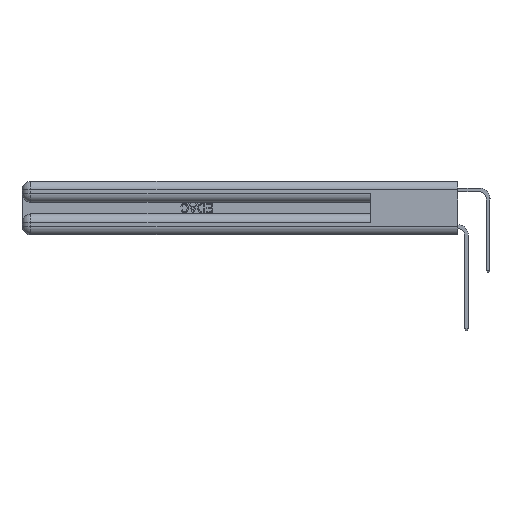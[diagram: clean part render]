
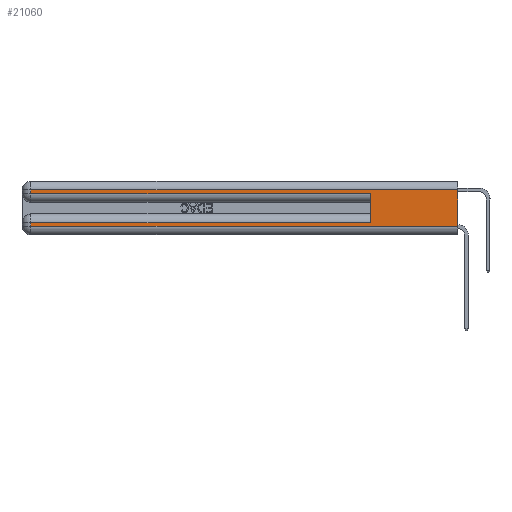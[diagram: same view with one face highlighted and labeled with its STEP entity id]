
A CAD part, left-side view. The second image highlights one B-rep face of the part: STEP entity #21060.
In plain terms, the highlighted planar face has unit normal (-1, 0, 0).
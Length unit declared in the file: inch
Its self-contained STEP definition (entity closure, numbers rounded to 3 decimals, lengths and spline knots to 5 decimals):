
#535 = DIRECTION ( 'NONE',  ( 0., 0., -1. ) ) ;
#800 = ORIENTED_EDGE ( 'NONE', *, *, #20794, .T. ) ;
#1014 = AXIS2_PLACEMENT_3D ( 'NONE', #16914, #11546, #22222 ) ;
#1233 = VECTOR ( 'NONE', #24987, 39.37008 ) ;
#1885 = ORIENTED_EDGE ( 'NONE', *, *, #12425, .F. ) ;
#2637 = VECTOR ( 'NONE', #28939, 39.37008 ) ;
#2693 = CARTESIAN_POINT ( 'NONE',  ( 0., 2.94, 0.06 ) ) ;
#4234 = CARTESIAN_POINT ( 'NONE',  ( 0., 0.6, 0.285 ) ) ;
#4418 = VERTEX_POINT ( 'NONE', #12762 ) ;
#4594 = LINE ( 'NONE', #8954, #20139 ) ;
#5728 = LINE ( 'NONE', #24723, #25001 ) ;
#6314 = LINE ( 'NONE', #26965, #32523 ) ;
#6561 = EDGE_LOOP ( 'NONE', ( #26309, #16931, #18086, #800, #1885, #12907, #27303, #20859 ) ) ;
#7468 = VERTEX_POINT ( 'NONE', #22239 ) ;
#8585 = LINE ( 'NONE', #22189, #1233 ) ;
#8954 = CARTESIAN_POINT ( 'NONE',  ( 0., 0., 0.085 ) ) ;
#10558 = CARTESIAN_POINT ( 'NONE',  ( 0., 2.94, 0.37 ) ) ;
#10589 = EDGE_CURVE ( 'NONE', #4418, #31251, #4594, .T. ) ;
#11228 = VERTEX_POINT ( 'NONE', #32108 ) ;
#11546 = DIRECTION ( 'NONE',  ( 1., 0., 0. ) ) ;
#12266 = EDGE_CURVE ( 'NONE', #26008, #15922, #5728, .T. ) ;
#12351 = DIRECTION ( 'NONE',  ( 0., -1., 0. ) ) ;
#12425 = EDGE_CURVE ( 'NONE', #4418, #27533, #8585, .T. ) ;
#12454 = EDGE_CURVE ( 'NONE', #26530, #11228, #28262, .T. ) ;
#12762 = CARTESIAN_POINT ( 'NONE',  ( 0., 0.6, 0.085 ) ) ;
#12907 = ORIENTED_EDGE ( 'NONE', *, *, #10589, .T. ) ;
#13736 = CARTESIAN_POINT ( 'NONE',  ( 0., 2.94, 0.085 ) ) ;
#13955 = LINE ( 'NONE', #19787, #21388 ) ;
#14292 = CARTESIAN_POINT ( 'NONE',  ( 0., 2.94, 0.31 ) ) ;
#14314 = DIRECTION ( 'NONE',  ( 0., 1., 0. ) ) ;
#14643 = CARTESIAN_POINT ( 'NONE',  ( 0., 0., 0.06 ) ) ;
#14763 = FACE_OUTER_BOUND ( 'NONE', #6561, .T. ) ;
#15922 = VERTEX_POINT ( 'NONE', #14292 ) ;
#16099 = LINE ( 'NONE', #22874, #22285 ) ;
#16914 = CARTESIAN_POINT ( 'NONE',  ( 0., 0., 0.37 ) ) ;
#16931 = ORIENTED_EDGE ( 'NONE', *, *, #12266, .T. ) ;
#17521 = EDGE_CURVE ( 'NONE', #15922, #7468, #26025, .T. ) ;
#18086 = ORIENTED_EDGE ( 'NONE', *, *, #17521, .T. ) ;
#18542 = DIRECTION ( 'NONE',  ( 0., -1., 0. ) ) ;
#19787 = CARTESIAN_POINT ( 'NONE',  ( 0., 0., 0.285 ) ) ;
#20139 = VECTOR ( 'NONE', #29909, 39.37008 ) ;
#20434 = VECTOR ( 'NONE', #12351, 39.37008 ) ;
#20794 = EDGE_CURVE ( 'NONE', #7468, #27533, #13955, .T. ) ;
#20859 = ORIENTED_EDGE ( 'NONE', *, *, #12454, .T. ) ;
#21060 = ADVANCED_FACE ( 'NONE', ( #14763 ), #27623, .F. ) ;
#21388 = VECTOR ( 'NONE', #18542, 39.37008 ) ;
#22189 = CARTESIAN_POINT ( 'NONE',  ( 0., 0.6, 0.145 ) ) ;
#22222 = DIRECTION ( 'NONE',  ( 0., 0., -1. ) ) ;
#22239 = CARTESIAN_POINT ( 'NONE',  ( 0., 2.94, 0.285 ) ) ;
#22285 = VECTOR ( 'NONE', #33312, 39.37008 ) ;
#22874 = CARTESIAN_POINT ( 'NONE',  ( 0., 0., 0.37 ) ) ;
#24723 = CARTESIAN_POINT ( 'NONE',  ( 0., 0., 0.31 ) ) ;
#24987 = DIRECTION ( 'NONE',  ( 0., 0., 1. ) ) ;
#25001 = VECTOR ( 'NONE', #14314, 39.37008 ) ;
#26008 = VERTEX_POINT ( 'NONE', #31810 ) ;
#26025 = LINE ( 'NONE', #10558, #2637 ) ;
#26309 = ORIENTED_EDGE ( 'NONE', *, *, #27735, .F. ) ;
#26530 = VERTEX_POINT ( 'NONE', #2693 ) ;
#26710 = EDGE_CURVE ( 'NONE', #31251, #26530, #6314, .T. ) ;
#26965 = CARTESIAN_POINT ( 'NONE',  ( 0., 2.94, 0.37 ) ) ;
#27303 = ORIENTED_EDGE ( 'NONE', *, *, #26710, .T. ) ;
#27533 = VERTEX_POINT ( 'NONE', #4234 ) ;
#27623 = PLANE ( 'NONE',  #1014 ) ;
#27735 = EDGE_CURVE ( 'NONE', #26008, #11228, #16099, .T. ) ;
#28262 = LINE ( 'NONE', #14643, #20434 ) ;
#28939 = DIRECTION ( 'NONE',  ( 0., 0., -1. ) ) ;
#29909 = DIRECTION ( 'NONE',  ( 0., 1., 0. ) ) ;
#31251 = VERTEX_POINT ( 'NONE', #13736 ) ;
#31810 = CARTESIAN_POINT ( 'NONE',  ( 0., 0., 0.31 ) ) ;
#32108 = CARTESIAN_POINT ( 'NONE',  ( 0., 0., 0.06 ) ) ;
#32523 = VECTOR ( 'NONE', #535, 39.37008 ) ;
#33312 = DIRECTION ( 'NONE',  ( 0., 0., -1. ) ) ;
